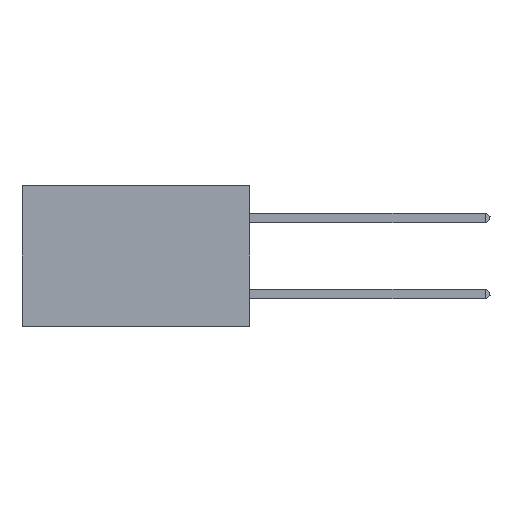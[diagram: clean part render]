
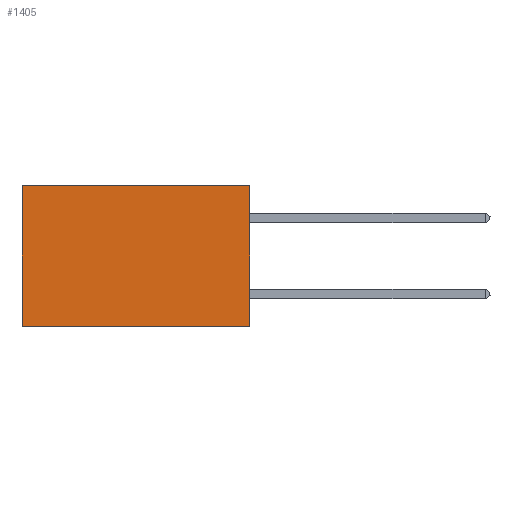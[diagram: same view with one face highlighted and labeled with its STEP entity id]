
A CAD part, left-side view. The second image highlights one B-rep face of the part: STEP entity #1405.
In plain terms, the highlighted planar face has unit normal (-1, 0, 0).
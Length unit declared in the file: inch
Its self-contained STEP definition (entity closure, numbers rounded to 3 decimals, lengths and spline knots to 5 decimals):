
#1009 = VERTEX_POINT ( 'NONE', #25575 ) ;
#1405 = ADVANCED_FACE ( 'NONE', ( #3449 ), #3679, .F. ) ;
#2702 = CARTESIAN_POINT ( 'NONE',  ( 0.2875, 0., 0. ) ) ;
#2953 = VECTOR ( 'NONE', #14641, 39.37008 ) ;
#3449 = FACE_OUTER_BOUND ( 'NONE', #21513, .T. ) ;
#3679 = PLANE ( 'NONE',  #31575 ) ;
#3747 = LINE ( 'NONE', #26815, #2953 ) ;
#5138 = EDGE_CURVE ( 'NONE', #9697, #31217, #12662, .T. ) ;
#8996 = CARTESIAN_POINT ( 'NONE',  ( 0.2875, 0., 0. ) ) ;
#9697 = VERTEX_POINT ( 'NONE', #8996 ) ;
#10021 = LINE ( 'NONE', #23642, #15860 ) ;
#10918 = LINE ( 'NONE', #12089, #30424 ) ;
#11052 = EDGE_CURVE ( 'NONE', #9697, #26622, #10918, .T. ) ;
#11753 = EDGE_CURVE ( 'NONE', #26622, #1009, #3747, .T. ) ;
#12089 = CARTESIAN_POINT ( 'NONE',  ( 0.2875, 0., 0. ) ) ;
#12662 = LINE ( 'NONE', #2702, #25718 ) ;
#13671 = CARTESIAN_POINT ( 'NONE',  ( 0.2875, 0., 0. ) ) ;
#14641 = DIRECTION ( 'NONE',  ( 0., 1., 0. ) ) ;
#15064 = DIRECTION ( 'NONE',  ( 0., 0., -1. ) ) ;
#15239 = ORIENTED_EDGE ( 'NONE', *, *, #23054, .T. ) ;
#15860 = VECTOR ( 'NONE', #28482, 39.37008 ) ;
#16237 = ORIENTED_EDGE ( 'NONE', *, *, #11052, .F. ) ;
#19854 = CARTESIAN_POINT ( 'NONE',  ( 0.2875, 0., -0.37 ) ) ;
#20205 = DIRECTION ( 'NONE',  ( 0., 1., 0. ) ) ;
#21173 = ORIENTED_EDGE ( 'NONE', *, *, #5138, .T. ) ;
#21513 = EDGE_LOOP ( 'NONE', ( #15239, #25051, #16237, #21173 ) ) ;
#23054 = EDGE_CURVE ( 'NONE', #31217, #1009, #10021, .T. ) ;
#23642 = CARTESIAN_POINT ( 'NONE',  ( 0.2875, 0.6, 0. ) ) ;
#25051 = ORIENTED_EDGE ( 'NONE', *, *, #11753, .F. ) ;
#25575 = CARTESIAN_POINT ( 'NONE',  ( 0.2875, 0.6, -0.37 ) ) ;
#25718 = VECTOR ( 'NONE', #20205, 39.37008 ) ;
#26622 = VERTEX_POINT ( 'NONE', #19854 ) ;
#26815 = CARTESIAN_POINT ( 'NONE',  ( 0.2875, 0., -0.37 ) ) ;
#28482 = DIRECTION ( 'NONE',  ( 0., 0., -1. ) ) ;
#29180 = DIRECTION ( 'NONE',  ( 0., 0., -1. ) ) ;
#29830 = CARTESIAN_POINT ( 'NONE',  ( 0.2875, 0.6, 0. ) ) ;
#30424 = VECTOR ( 'NONE', #29180, 39.37008 ) ;
#31217 = VERTEX_POINT ( 'NONE', #29830 ) ;
#31575 = AXIS2_PLACEMENT_3D ( 'NONE', #13671, #32027, #15064 ) ;
#32027 = DIRECTION ( 'NONE',  ( 1., 0., 0. ) ) ;
